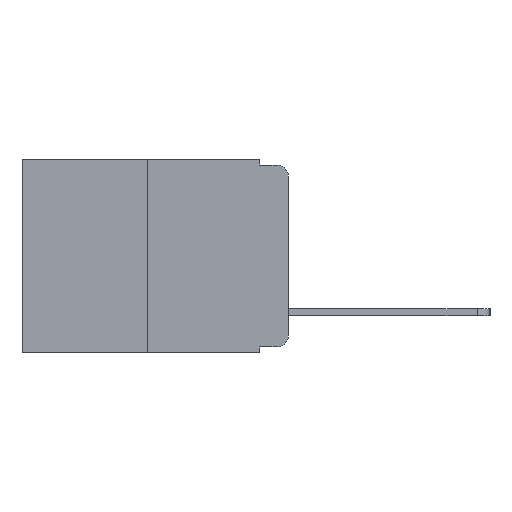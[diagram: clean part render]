
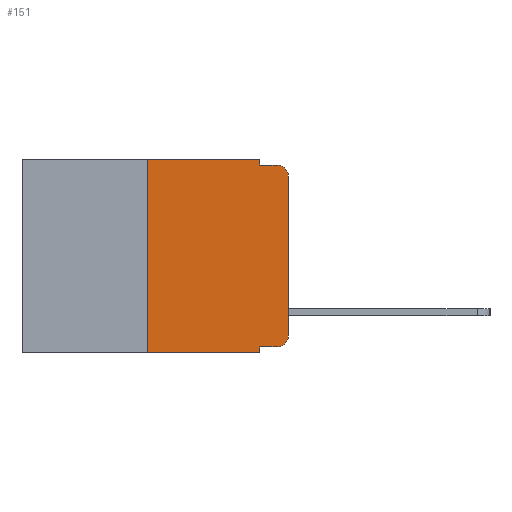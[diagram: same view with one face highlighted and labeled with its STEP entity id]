
A CAD part, left-side view. The second image highlights one B-rep face of the part: STEP entity #151.
In plain terms, the highlighted planar face has unit normal (-1, 0, 0).
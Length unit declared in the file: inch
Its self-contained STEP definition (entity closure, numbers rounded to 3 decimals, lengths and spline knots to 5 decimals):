
#19 = EDGE_CURVE ( 'NONE', #6691, #10626, #11475, .T. ) ;
#25 = EDGE_CURVE ( 'NONE', #13941, #6691, #17971, .T. ) ;
#29 = EDGE_CURVE ( 'NONE', #7083, #6158, #2780, .T. ) ;
#59 = EDGE_CURVE ( 'NONE', #11740, #18361, #13958, .T. ) ;
#66 = EDGE_CURVE ( 'NONE', #11740, #4840, #17135, .T. ) ;
#135 = EDGE_CURVE ( 'NONE', #4840, #1143, #12589, .T. ) ;
#151 = ADVANCED_FACE ( 'NONE', ( #3584 ), #7166, .F. ) ;
#464 = AXIS2_PLACEMENT_3D ( 'NONE', #16533, #8047, #17893 ) ;
#1132 = VECTOR ( 'NONE', #9004, 39.37008 ) ;
#1143 = VERTEX_POINT ( 'NONE', #3625 ) ;
#1532 = CARTESIAN_POINT ( 'NONE',  ( 0., 0.25, 0. ) ) ;
#1600 = DIRECTION ( 'NONE',  ( 0., 0., -1. ) ) ;
#1856 = CARTESIAN_POINT ( 'NONE',  ( 0., 0., 0. ) ) ;
#2557 = LINE ( 'NONE', #1856, #17395 ) ;
#2577 = CARTESIAN_POINT ( 'NONE',  ( 0., 0.25, -0.343 ) ) ;
#2780 = LINE ( 'NONE', #6656, #14813 ) ;
#3275 = ORIENTED_EDGE ( 'NONE', *, *, #16842, .T. ) ;
#3314 = ORIENTED_EDGE ( 'NONE', *, *, #17543, .T. ) ;
#3422 = ORIENTED_EDGE ( 'NONE', *, *, #19, .F. ) ;
#3428 = ORIENTED_EDGE ( 'NONE', *, *, #25, .F. ) ;
#3456 = ORIENTED_EDGE ( 'NONE', *, *, #14580, .F. ) ;
#3584 = FACE_OUTER_BOUND ( 'NONE', #5815, .T. ) ;
#3618 = DIRECTION ( 'NONE',  ( 0., 0., 1. ) ) ;
#3625 = CARTESIAN_POINT ( 'NONE',  ( 0., 0., -0.313 ) ) ;
#3703 = ORIENTED_EDGE ( 'NONE', *, *, #29, .F. ) ;
#3776 = ORIENTED_EDGE ( 'NONE', *, *, #17081, .T. ) ;
#3781 = CARTESIAN_POINT ( 'NONE',  ( 0., 0.051, -0.01 ) ) ;
#3814 = ORIENTED_EDGE ( 'NONE', *, *, #59, .F. ) ;
#3884 = CARTESIAN_POINT ( 'NONE',  ( 0., 0.473, 0. ) ) ;
#3962 = ORIENTED_EDGE ( 'NONE', *, *, #66, .T. ) ;
#4119 = VERTEX_POINT ( 'NONE', #10942 ) ;
#4242 = LINE ( 'NONE', #3884, #15159 ) ;
#4463 = CARTESIAN_POINT ( 'NONE',  ( 0., 0.051, -0.333 ) ) ;
#4578 = AXIS2_PLACEMENT_3D ( 'NONE', #14363, #14511, #13076 ) ;
#4778 = CARTESIAN_POINT ( 'NONE',  ( 0., 0.051, -0.01 ) ) ;
#4840 = VERTEX_POINT ( 'NONE', #5022 ) ;
#5022 = CARTESIAN_POINT ( 'NONE',  ( 0., 0.02, -0.333 ) ) ;
#5299 = DIRECTION ( 'NONE',  ( 1., 0., 0. ) ) ;
#5501 = DIRECTION ( 'NONE',  ( 0., -1., 0. ) ) ;
#5521 = DIRECTION ( 'NONE',  ( 0., -1., 0. ) ) ;
#5675 = CARTESIAN_POINT ( 'NONE',  ( 0., 0.473, -0.343 ) ) ;
#5773 = CARTESIAN_POINT ( 'NONE',  ( 0., 0.051, 0. ) ) ;
#5815 = EDGE_LOOP ( 'NONE', ( #3275, #3314, #3422, #3428, #3456, #3703, #3776, #3814, #3962, #6526 ) ) ;
#6158 = VERTEX_POINT ( 'NONE', #1532 ) ;
#6526 = ORIENTED_EDGE ( 'NONE', *, *, #135, .T. ) ;
#6591 = DIRECTION ( 'NONE',  ( 0., 0., -1. ) ) ;
#6656 = CARTESIAN_POINT ( 'NONE',  ( 0., 0.25, 0. ) ) ;
#6691 = VERTEX_POINT ( 'NONE', #4778 ) ;
#7083 = VERTEX_POINT ( 'NONE', #2577 ) ;
#7125 = VECTOR ( 'NONE', #11675, 39.37008 ) ;
#7166 = PLANE ( 'NONE',  #10713 ) ;
#7575 = VECTOR ( 'NONE', #5501, 39.37008 ) ;
#8047 = DIRECTION ( 'NONE',  ( -1., 0., 0. ) ) ;
#8134 = CARTESIAN_POINT ( 'NONE',  ( 0., 0.051, -0.343 ) ) ;
#8358 = DIRECTION ( 'NONE',  ( 0., 0., -1. ) ) ;
#9004 = DIRECTION ( 'NONE',  ( 0., -1., 0. ) ) ;
#9230 = CARTESIAN_POINT ( 'NONE',  ( 0., 0.051, -0.333 ) ) ;
#10004 = CARTESIAN_POINT ( 'NONE',  ( 0., 0.051, 0. ) ) ;
#10203 = CIRCLE ( 'NONE', #464, 0.02 ) ;
#10574 = VECTOR ( 'NONE', #1600, 39.37008 ) ;
#10626 = VERTEX_POINT ( 'NONE', #11139 ) ;
#10713 = AXIS2_PLACEMENT_3D ( 'NONE', #14345, #5299, #8358 ) ;
#10942 = CARTESIAN_POINT ( 'NONE',  ( 0., 0., -0.03 ) ) ;
#11139 = CARTESIAN_POINT ( 'NONE',  ( 0., 0.02, -0.01 ) ) ;
#11475 = LINE ( 'NONE', #3781, #7575 ) ;
#11675 = DIRECTION ( 'NONE',  ( 0., -1., 0. ) ) ;
#11740 = VERTEX_POINT ( 'NONE', #4463 ) ;
#12589 = CIRCLE ( 'NONE', #4578, 0.02 ) ;
#13076 = DIRECTION ( 'NONE',  ( 0., 0., -1. ) ) ;
#13941 = VERTEX_POINT ( 'NONE', #10004 ) ;
#13958 = LINE ( 'NONE', #14218, #10574 ) ;
#14218 = CARTESIAN_POINT ( 'NONE',  ( 0., 0.051, 0. ) ) ;
#14345 = CARTESIAN_POINT ( 'NONE',  ( 0., 0.473, 0. ) ) ;
#14363 = CARTESIAN_POINT ( 'NONE',  ( 0., 0.02, -0.313 ) ) ;
#14398 = VECTOR ( 'NONE', #6591, 39.37008 ) ;
#14511 = DIRECTION ( 'NONE',  ( -1., 0., 0. ) ) ;
#14580 = EDGE_CURVE ( 'NONE', #6158, #13941, #4242, .T. ) ;
#14813 = VECTOR ( 'NONE', #18052, 39.37008 ) ;
#15159 = VECTOR ( 'NONE', #5521, 39.37008 ) ;
#16533 = CARTESIAN_POINT ( 'NONE',  ( 0., 0.02, -0.03 ) ) ;
#16842 = EDGE_CURVE ( 'NONE', #1143, #4119, #2557, .T. ) ;
#17081 = EDGE_CURVE ( 'NONE', #7083, #18361, #18434, .T. ) ;
#17135 = LINE ( 'NONE', #9230, #1132 ) ;
#17395 = VECTOR ( 'NONE', #3618, 39.37008 ) ;
#17543 = EDGE_CURVE ( 'NONE', #4119, #10626, #10203, .T. ) ;
#17893 = DIRECTION ( 'NONE',  ( 0., 0., -1. ) ) ;
#17971 = LINE ( 'NONE', #5773, #14398 ) ;
#18052 = DIRECTION ( 'NONE',  ( 0., 0., 1. ) ) ;
#18361 = VERTEX_POINT ( 'NONE', #8134 ) ;
#18434 = LINE ( 'NONE', #5675, #7125 ) ;
